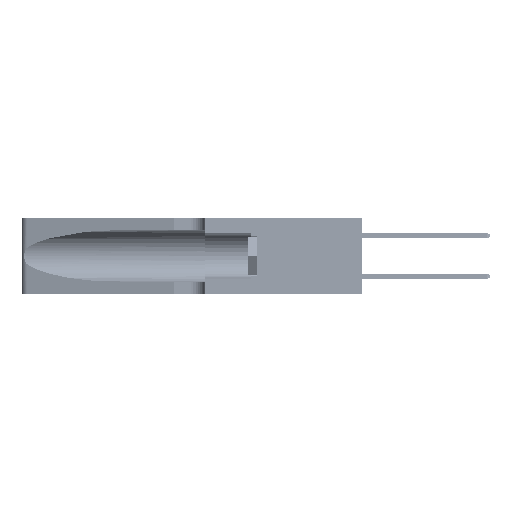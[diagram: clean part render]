
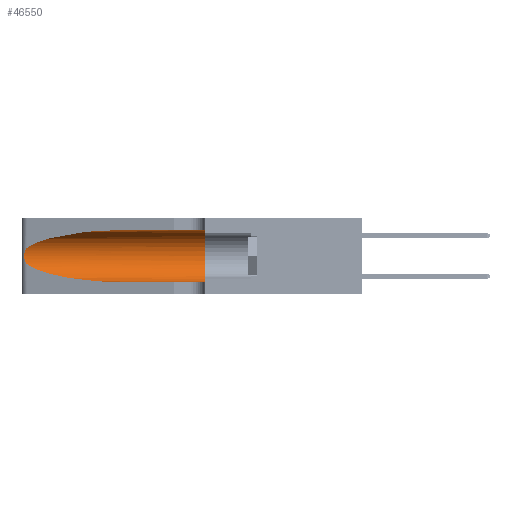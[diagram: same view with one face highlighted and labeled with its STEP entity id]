
A CAD part, left-side view. The second image highlights one B-rep face of the part: STEP entity #46550.
In plain terms, the highlighted cylindrical face has radius 3.308 mm (diameter 6.617 mm), a partial arc.
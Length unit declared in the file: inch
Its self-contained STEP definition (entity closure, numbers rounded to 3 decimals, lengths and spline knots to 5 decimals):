
#1028 = VERTEX_POINT ( 'NONE', #43649 ) ;
#1413 = CARTESIAN_POINT ( 'NONE',  ( 0.1305, 0.35, 0.31525 ) ) ;
#2025 = CIRCLE ( 'NONE', #45687, 0.13025 ) ;
#2803 = CARTESIAN_POINT ( 'NONE',  ( 0.1305, 1.61858, 0.185 ) ) ;
#2840 = CARTESIAN_POINT ( 'NONE',  ( 0.18966, 0.96281, 0.05475 ) ) ;
#3868 = CARTESIAN_POINT ( 'NONE',  ( 0.26017, 1.23833, 0.17102 ) ) ;
#4728 = CARTESIAN_POINT ( 'NONE',  ( 0.25487, 1.22718, 0.22369 ) ) ;
#5439 = VERTEX_POINT ( 'NONE', #31654 ) ;
#5471 = CARTESIAN_POINT ( 'NONE',  ( 0.1305, 0.35, 0.185 ) ) ;
#7018 = DIRECTION ( 'NONE',  ( 0., 0., -1. ) ) ;
#7896 = CARTESIAN_POINT ( 'NONE',  ( 0.25487, 1.22718, 0.22369 ) ) ;
#8065 = CARTESIAN_POINT ( 'NONE',  ( 0.25789, 1.23486, 0.15765 ) ) ;
#8337 = VERTEX_POINT ( 'NONE', #25987 ) ;
#9346 = VECTOR ( 'NONE', #42934, 39.37008 ) ;
#9402 = EDGE_CURVE ( 'NONE', #31078, #34409, #42300, .T. ) ;
#9679 = DIRECTION ( 'NONE',  ( 0., 0., 1. ) ) ;
#9905 = EDGE_CURVE ( 'NONE', #31078, #8337, #11455, .T. ) ;
#9924 = CARTESIAN_POINT ( 'NONE',  ( 0.1305, 1.61858, 0.31525 ) ) ;
#10893 = CARTESIAN_POINT ( 'NONE',  ( 0.1305, 1.61858, 0.05475 ) ) ;
#11105 = ORIENTED_EDGE ( 'NONE', *, *, #18969, .F. ) ;
#11394 = FACE_OUTER_BOUND ( 'NONE', #27768, .T. ) ;
#11455 =( BOUNDED_CURVE ( )  B_SPLINE_CURVE ( 3, ( #33526, #17073, #29566, #4728 ),
 .UNSPECIFIED., .F., .F. ) 
 B_SPLINE_CURVE_WITH_KNOTS ( ( 4, 4 ),
 ( 1.5708, 2.84003 ),
 .UNSPECIFIED. ) 
 CURVE ( )  GEOMETRIC_REPRESENTATION_ITEM ( )  RATIONAL_B_SPLINE_CURVE ( ( 1., 0.87, 0.87, 1. ) ) 
 REPRESENTATION_ITEM ( '' )  );
#12188 = CARTESIAN_POINT ( 'NONE',  ( 0.25555, 1.22993, 0.14849 ) ) ;
#13870 = EDGE_CURVE ( 'NONE', #1028, #25448, #49665, .T. ) ;
#16026 = CARTESIAN_POINT ( 'NONE',  ( 0.25555, 1.22994, 0.2215 ) ) ;
#17073 = CARTESIAN_POINT ( 'NONE',  ( 0.18966, 0.96281, 0.31525 ) ) ;
#18969 = EDGE_CURVE ( 'NONE', #34409, #25448, #2025, .T. ) ;
#19358 = CARTESIAN_POINT ( 'NONE',  ( 0.2373, 1.15595, 0.08982 ) ) ;
#20348 = CARTESIAN_POINT ( 'NONE',  ( 0.25787, 1.23484, 0.2124 ) ) ;
#23160 = EDGE_CURVE ( 'NONE', #8337, #5439, #44228, .T. ) ;
#24328 = EDGE_CURVE ( 'NONE', #5439, #1028, #47511, .T. ) ;
#24505 = CARTESIAN_POINT ( 'NONE',  ( 0.26018, 1.23835, 0.19895 ) ) ;
#25448 = VERTEX_POINT ( 'NONE', #32934 ) ;
#25987 = CARTESIAN_POINT ( 'NONE',  ( 0.25487, 1.22718, 0.22369 ) ) ;
#27514 = DIRECTION ( 'NONE',  ( 0., -1., 0. ) ) ;
#27764 = VECTOR ( 'NONE', #27514, 39.37008 ) ;
#27768 = EDGE_LOOP ( 'NONE', ( #52005, #53471, #50964, #48926, #11105, #40114 ) ) ;
#28689 = CARTESIAN_POINT ( 'NONE',  ( 0.26075, 1.23896, 0.178 ) ) ;
#29566 = CARTESIAN_POINT ( 'NONE',  ( 0.2373, 1.15595, 0.28018 ) ) ;
#31078 = VERTEX_POINT ( 'NONE', #41904 ) ;
#31654 = CARTESIAN_POINT ( 'NONE',  ( 0.25487, 1.22718, 0.14631 ) ) ;
#31801 = DIRECTION ( 'NONE',  ( 0., -1., 0. ) ) ;
#31842 = CARTESIAN_POINT ( 'NONE',  ( 0.1305, 0.72297, 0.05475 ) ) ;
#32840 = CARTESIAN_POINT ( 'NONE',  ( 0.25856, 1.23593, 0.16098 ) ) ;
#32934 = CARTESIAN_POINT ( 'NONE',  ( 0.1305, 0.35, 0.05475 ) ) ;
#33526 = CARTESIAN_POINT ( 'NONE',  ( 0.1305, 0.72297, 0.31525 ) ) ;
#34409 = VERTEX_POINT ( 'NONE', #1413 ) ;
#34422 = DIRECTION ( 'NONE',  ( 0., 1., 0. ) ) ;
#36984 = CARTESIAN_POINT ( 'NONE',  ( 0.25639, 1.23186, 0.15144 ) ) ;
#40114 = ORIENTED_EDGE ( 'NONE', *, *, #9402, .F. ) ;
#40867 = AXIS2_PLACEMENT_3D ( 'NONE', #2803, #31801, #7018 ) ;
#41108 = CARTESIAN_POINT ( 'NONE',  ( 0.25487, 1.22718, 0.14631 ) ) ;
#41904 = CARTESIAN_POINT ( 'NONE',  ( 0.1305, 0.72297, 0.31525 ) ) ;
#42300 = LINE ( 'NONE', #9924, #9346 ) ;
#42934 = DIRECTION ( 'NONE',  ( 0., -1., 0. ) ) ;
#43036 = CYLINDRICAL_SURFACE ( 'NONE', #40867, 0.13025 ) ;
#43649 = CARTESIAN_POINT ( 'NONE',  ( 0.1305, 0.72297, 0.05475 ) ) ;
#44228 = B_SPLINE_CURVE_WITH_KNOTS ( 'NONE', 3,
 ( #7896, #16026, #45078, #20348, #49226, #24505, #53317, #28689, #3868, #32840, #8065, #36984, #12188, #41108 ),
 .UNSPECIFIED., .F., .F.,
 ( 4, 2, 2, 2, 2, 2, 4 ),
 ( 0., 0.00027, 0.00053, 0.00107, 0.0016, 0.00187, 0.00214 ),
 .UNSPECIFIED. ) ;
#45078 = CARTESIAN_POINT ( 'NONE',  ( 0.25639, 1.23184, 0.21858 ) ) ;
#45687 = AXIS2_PLACEMENT_3D ( 'NONE', #5471, #34422, #9679 ) ;
#46550 = ADVANCED_FACE ( 'NONE', ( #11394 ), #43036, .F. ) ;
#47511 =( BOUNDED_CURVE ( )  B_SPLINE_CURVE ( 3, ( #52311, #19358, #2840, #31842 ),
 .UNSPECIFIED., .F., .T. ) 
 B_SPLINE_CURVE_WITH_KNOTS ( ( 4, 4 ),
 ( 3.44316, 4.71239 ),
 .UNSPECIFIED. ) 
 CURVE ( )  GEOMETRIC_REPRESENTATION_ITEM ( )  RATIONAL_B_SPLINE_CURVE ( ( 1., 0.87, 0.87, 1. ) ) 
 REPRESENTATION_ITEM ( '' )  );
#48926 = ORIENTED_EDGE ( 'NONE', *, *, #13870, .T. ) ;
#49226 = CARTESIAN_POINT ( 'NONE',  ( 0.25854, 1.2359, 0.20912 ) ) ;
#49665 = LINE ( 'NONE', #10893, #27764 ) ;
#50964 = ORIENTED_EDGE ( 'NONE', *, *, #24328, .T. ) ;
#52005 = ORIENTED_EDGE ( 'NONE', *, *, #9905, .T. ) ;
#52311 = CARTESIAN_POINT ( 'NONE',  ( 0.25487, 1.22718, 0.14631 ) ) ;
#53317 = CARTESIAN_POINT ( 'NONE',  ( 0.26075, 1.23896, 0.19203 ) ) ;
#53471 = ORIENTED_EDGE ( 'NONE', *, *, #23160, .T. ) ;
